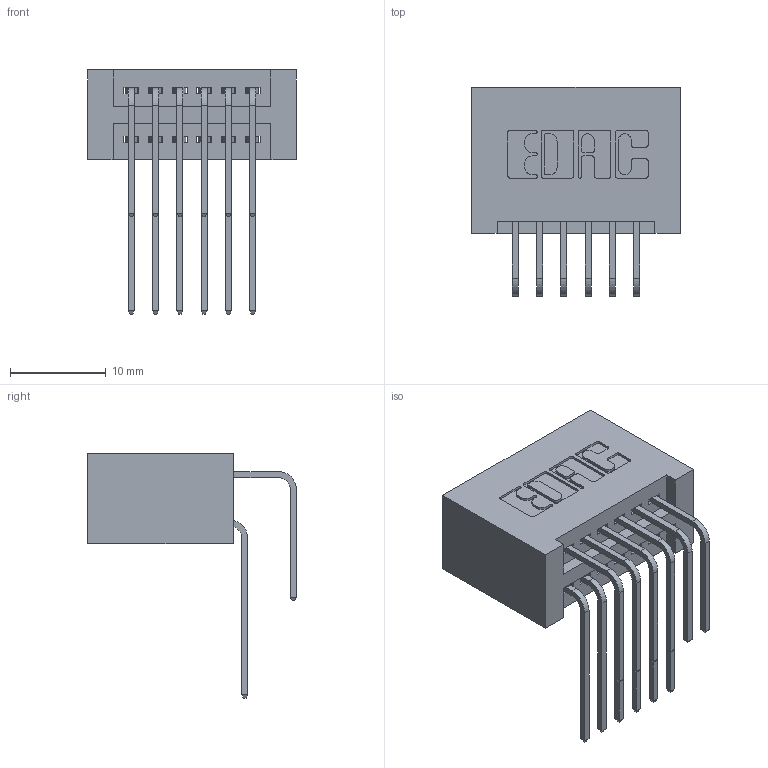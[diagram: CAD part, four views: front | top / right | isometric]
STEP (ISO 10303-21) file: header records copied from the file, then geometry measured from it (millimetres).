
FILE_DESCRIPTION (( 'STEP AP203' ), '1' );
FILE_NAME ('395-012-558-201.STEP', '2018-11-05T19:44:49', ( '' ), ( '' ), 'SwSTEP 2.0', 'SolidWorks 2016', '' );
FILE_SCHEMA (( 'CONFIG_CONTROL_DESIGN' ));
Length unit declared in the file: inch
Products named in the file (4): 345-292-001_558 Tail - 2; 345-292-001_558 559 Tail - 1; 345 Part_No Mounting Lugs; 395-012-558-201
Assembly tree (13 placements, depth 2):
  395-012-558-201
    345 Part_No Mounting Lugs
    345-292-001_558 559 Tail - 1  x6
    345-292-001_558 Tail - 2  x6
Bounding box: 21.84 x 21.83 x 25.53 mm (x, y, z)
Volume: 2472.9 mm3; surface area: 3586.9 mm2
Topology: 13 solids, 13 shells, 742 faces, 2177 edges, 1434 vertices
Faces by surface type: plane 496, cylinder 246
Entity records: 10929 total; most frequent: CARTESIAN_POINT 1911, ORIENTED_EDGE 1794, DIRECTION 1697, EDGE_CURVE 897, LINE 709, VECTOR 709, VERTEX_POINT 594, AXIS2_PLACEMENT_3D 494
